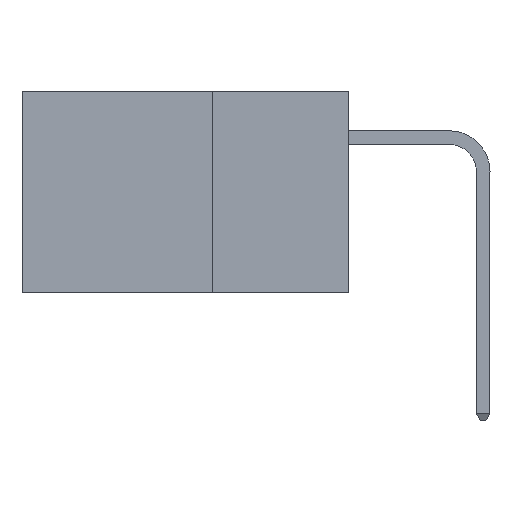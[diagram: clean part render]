
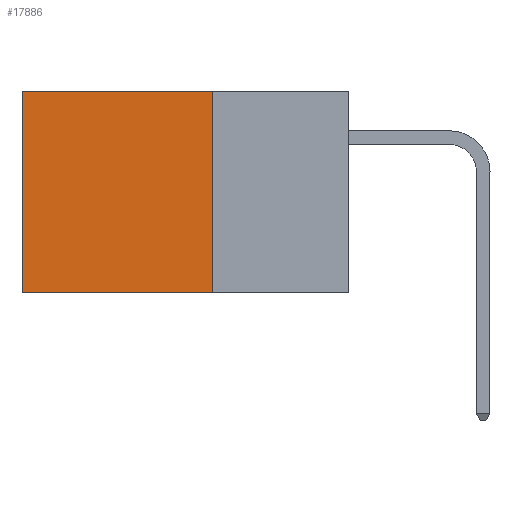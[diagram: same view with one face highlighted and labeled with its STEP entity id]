
A CAD part, left-side view. The second image highlights one B-rep face of the part: STEP entity #17886.
In plain terms, the highlighted planar face has unit normal (-1, 0, 0).
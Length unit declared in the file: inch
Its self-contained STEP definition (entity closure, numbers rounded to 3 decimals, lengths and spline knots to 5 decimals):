
#1362 = ORIENTED_EDGE ( 'NONE', *, *, #26078, .T. ) ;
#1833 = DIRECTION ( 'NONE',  ( 0., 1., 0. ) ) ;
#2088 = VERTEX_POINT ( 'NONE', #33120 ) ;
#5174 = ORIENTED_EDGE ( 'NONE', *, *, #27790, .T. ) ;
#5338 = FACE_OUTER_BOUND ( 'NONE', #34975, .T. ) ;
#5540 = LINE ( 'NONE', #33892, #5640 ) ;
#5640 = VECTOR ( 'NONE', #9068, 39.37008 ) ;
#8323 = VERTEX_POINT ( 'NONE', #30275 ) ;
#8983 = VECTOR ( 'NONE', #24507, 39.37008 ) ;
#9068 = DIRECTION ( 'NONE',  ( 0., 0., -1. ) ) ;
#9127 = VECTOR ( 'NONE', #1833, 39.37008 ) ;
#9234 = LINE ( 'NONE', #15841, #9127 ) ;
#10466 = DIRECTION ( 'NONE',  ( 1., 0., 0. ) ) ;
#10577 = DIRECTION ( 'NONE',  ( 0., 0., -1. ) ) ;
#11633 = EDGE_CURVE ( 'NONE', #17662, #28683, #23698, .T. ) ;
#15841 = CARTESIAN_POINT ( 'NONE',  ( 0.2875, 0.25, 0. ) ) ;
#17662 = VERTEX_POINT ( 'NONE', #34320 ) ;
#17886 = ADVANCED_FACE ( 'NONE', ( #5338 ), #27161, .F. ) ;
#20177 = LINE ( 'NONE', #32734, #8983 ) ;
#22227 = CARTESIAN_POINT ( 'NONE',  ( 0.2875, 0.6, -0.37 ) ) ;
#23665 = VECTOR ( 'NONE', #34723, 39.37008 ) ;
#23698 = LINE ( 'NONE', #34800, #23665 ) ;
#24379 = CARTESIAN_POINT ( 'NONE',  ( 0.2875, 0.25, 0. ) ) ;
#24507 = DIRECTION ( 'NONE',  ( 0., 0., -1. ) ) ;
#25121 = AXIS2_PLACEMENT_3D ( 'NONE', #24379, #10466, #10577 ) ;
#25241 = ORIENTED_EDGE ( 'NONE', *, *, #11633, .F. ) ;
#26078 = EDGE_CURVE ( 'NONE', #2088, #28683, #20177, .T. ) ;
#27161 = PLANE ( 'NONE',  #25121 ) ;
#27790 = EDGE_CURVE ( 'NONE', #8323, #2088, #9234, .T. ) ;
#28683 = VERTEX_POINT ( 'NONE', #22227 ) ;
#30275 = CARTESIAN_POINT ( 'NONE',  ( 0.2875, 0.25, 0. ) ) ;
#31286 = ORIENTED_EDGE ( 'NONE', *, *, #32661, .F. ) ;
#32661 = EDGE_CURVE ( 'NONE', #8323, #17662, #5540, .T. ) ;
#32734 = CARTESIAN_POINT ( 'NONE',  ( 0.2875, 0.6, 0. ) ) ;
#33120 = CARTESIAN_POINT ( 'NONE',  ( 0.2875, 0.6, 0. ) ) ;
#33892 = CARTESIAN_POINT ( 'NONE',  ( 0.2875, 0.25, 0. ) ) ;
#34320 = CARTESIAN_POINT ( 'NONE',  ( 0.2875, 0.25, -0.37 ) ) ;
#34723 = DIRECTION ( 'NONE',  ( 0., 1., 0. ) ) ;
#34800 = CARTESIAN_POINT ( 'NONE',  ( 0.2875, 0.25, -0.37 ) ) ;
#34975 = EDGE_LOOP ( 'NONE', ( #1362, #25241, #31286, #5174 ) ) ;
